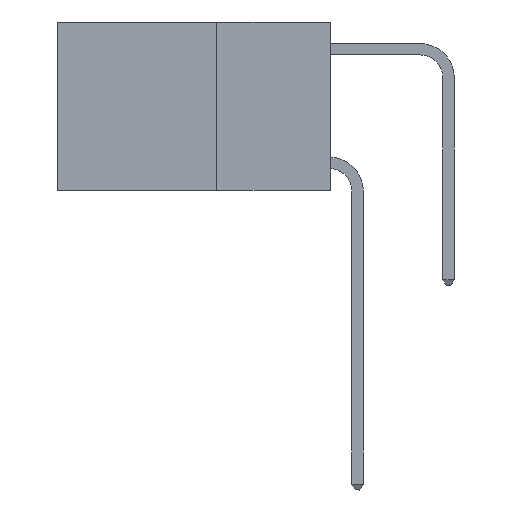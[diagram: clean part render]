
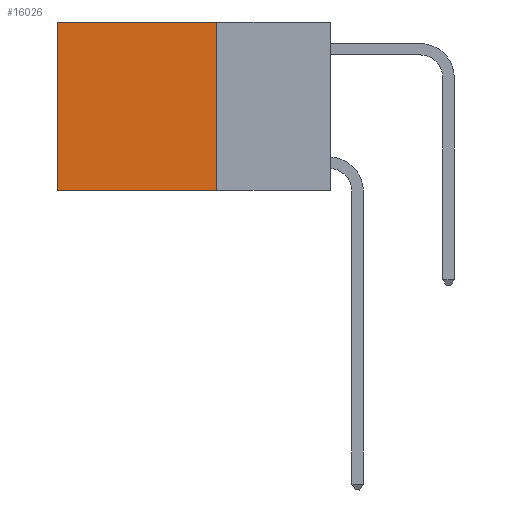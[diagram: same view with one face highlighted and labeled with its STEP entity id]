
A CAD part, left-side view. The second image highlights one B-rep face of the part: STEP entity #16026.
In plain terms, the highlighted planar face has unit normal (-1, 0, 0).
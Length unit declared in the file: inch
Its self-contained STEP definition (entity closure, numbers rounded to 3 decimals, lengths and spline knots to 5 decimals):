
#134 = DIRECTION ( 'NONE',  ( 0., 0., -1. ) ) ;
#776 = AXIS2_PLACEMENT_3D ( 'NONE', #18861, #10360, #134 ) ;
#1595 = DIRECTION ( 'NONE',  ( 0., 0., -1. ) ) ;
#2007 = ORIENTED_EDGE ( 'NONE', *, *, #17645, .F. ) ;
#2644 = FACE_OUTER_BOUND ( 'NONE', #3561, .T. ) ;
#3131 = CARTESIAN_POINT ( 'NONE',  ( 0.2625, 0.25, -0.37 ) ) ;
#3561 = EDGE_LOOP ( 'NONE', ( #7936, #2007, #13586, #14293 ) ) ;
#3757 = CARTESIAN_POINT ( 'NONE',  ( 0.2625, 0.6, -0.37 ) ) ;
#4728 = EDGE_CURVE ( 'NONE', #11638, #13345, #9249, .T. ) ;
#5214 = VECTOR ( 'NONE', #10227, 39.37008 ) ;
#6835 = CARTESIAN_POINT ( 'NONE',  ( 0.2625, 0.25, 0. ) ) ;
#6977 = PLANE ( 'NONE',  #776 ) ;
#7936 = ORIENTED_EDGE ( 'NONE', *, *, #4728, .T. ) ;
#9249 = LINE ( 'NONE', #13564, #17244 ) ;
#9772 = LINE ( 'NONE', #6835, #5214 ) ;
#10227 = DIRECTION ( 'NONE',  ( 0., 1., 0. ) ) ;
#10360 = DIRECTION ( 'NONE',  ( 1., 0., 0. ) ) ;
#11638 = VERTEX_POINT ( 'NONE', #18164 ) ;
#11940 = EDGE_CURVE ( 'NONE', #21150, #11638, #9772, .T. ) ;
#12386 = DIRECTION ( 'NONE',  ( 0., 1., 0. ) ) ;
#12818 = VECTOR ( 'NONE', #16131, 39.37008 ) ;
#13345 = VERTEX_POINT ( 'NONE', #3757 ) ;
#13361 = LINE ( 'NONE', #14408, #12818 ) ;
#13564 = CARTESIAN_POINT ( 'NONE',  ( 0.2625, 0.6, 0. ) ) ;
#13586 = ORIENTED_EDGE ( 'NONE', *, *, #18293, .F. ) ;
#14293 = ORIENTED_EDGE ( 'NONE', *, *, #11940, .T. ) ;
#14408 = CARTESIAN_POINT ( 'NONE',  ( 0.2625, 0.25, 0. ) ) ;
#14732 = CARTESIAN_POINT ( 'NONE',  ( 0.2625, 0.25, 0. ) ) ;
#16026 = ADVANCED_FACE ( 'NONE', ( #2644 ), #6977, .F. ) ;
#16131 = DIRECTION ( 'NONE',  ( 0., 0., -1. ) ) ;
#17244 = VECTOR ( 'NONE', #1595, 39.37008 ) ;
#17645 = EDGE_CURVE ( 'NONE', #19586, #13345, #20282, .T. ) ;
#18164 = CARTESIAN_POINT ( 'NONE',  ( 0.2625, 0.6, 0. ) ) ;
#18293 = EDGE_CURVE ( 'NONE', #21150, #19586, #13361, .T. ) ;
#18861 = CARTESIAN_POINT ( 'NONE',  ( 0.2625, 0.25, 0. ) ) ;
#19586 = VERTEX_POINT ( 'NONE', #3131 ) ;
#20282 = LINE ( 'NONE', #20841, #20796 ) ;
#20796 = VECTOR ( 'NONE', #12386, 39.37008 ) ;
#20841 = CARTESIAN_POINT ( 'NONE',  ( 0.2625, 0.25, -0.37 ) ) ;
#21150 = VERTEX_POINT ( 'NONE', #14732 ) ;
